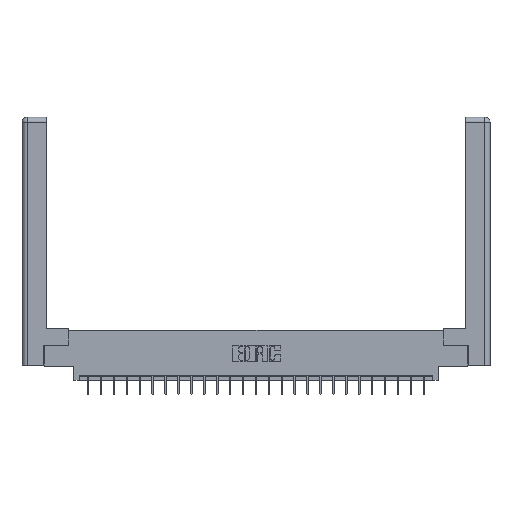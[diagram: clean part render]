
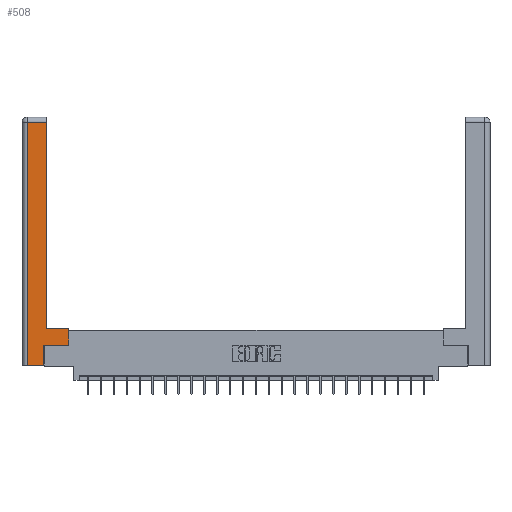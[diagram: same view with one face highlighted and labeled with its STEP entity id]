
A CAD part, top view. The second image highlights one B-rep face of the part: STEP entity #508.
In plain terms, the highlighted planar face has unit normal (0, 0, 1).
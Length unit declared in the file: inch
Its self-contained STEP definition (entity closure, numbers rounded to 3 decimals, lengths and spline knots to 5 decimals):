
#140 = FACE_OUTER_BOUND ( 'NONE', #25302, .T. ) ;
#165 = DIRECTION ( 'NONE',  ( 0., 1., 0. ) ) ;
#508 = ADVANCED_FACE ( 'NONE', ( #140 ), #7640, .F. ) ;
#1192 = ORIENTED_EDGE ( 'NONE', *, *, #4811, .T. ) ;
#1405 = DIRECTION ( 'NONE',  ( -1., 0., 0. ) ) ;
#1437 = ORIENTED_EDGE ( 'NONE', *, *, #23407, .T. ) ;
#1975 = LINE ( 'NONE', #7337, #19081 ) ;
#2334 = CARTESIAN_POINT ( 'NONE',  ( 0.0615, 0., 0. ) ) ;
#3073 = CARTESIAN_POINT ( 'NONE',  ( 0.295, 0.45, 0. ) ) ;
#4093 = CARTESIAN_POINT ( 'NONE',  ( 0.265, 0.245, 0. ) ) ;
#4225 = DIRECTION ( 'NONE',  ( 0., -1., 0. ) ) ;
#4312 = VERTEX_POINT ( 'NONE', #3073 ) ;
#4638 = VECTOR ( 'NONE', #24363, 39.37008 ) ;
#4811 = EDGE_CURVE ( 'NONE', #12248, #4312, #20631, .T. ) ;
#5860 = VECTOR ( 'NONE', #4225, 39.37008 ) ;
#6681 = ORIENTED_EDGE ( 'NONE', *, *, #22817, .T. ) ;
#6723 = VERTEX_POINT ( 'NONE', #22318 ) ;
#7089 = ORIENTED_EDGE ( 'NONE', *, *, #25089, .T. ) ;
#7107 = ORIENTED_EDGE ( 'NONE', *, *, #20207, .T. ) ;
#7214 = ORIENTED_EDGE ( 'NONE', *, *, #18998, .T. ) ;
#7253 = VECTOR ( 'NONE', #165, 39.37008 ) ;
#7297 = VECTOR ( 'NONE', #23084, 39.37008 ) ;
#7337 = CARTESIAN_POINT ( 'NONE',  ( 0.0615, 2.94, 0. ) ) ;
#7465 = CARTESIAN_POINT ( 'NONE',  ( 0.0615, 2.94, 0. ) ) ;
#7640 = PLANE ( 'NONE',  #12388 ) ;
#7835 = DIRECTION ( 'NONE',  ( 1., 0., 0. ) ) ;
#10400 = VERTEX_POINT ( 'NONE', #14519 ) ;
#10603 = VECTOR ( 'NONE', #7835, 39.37008 ) ;
#11315 = LINE ( 'NONE', #18001, #7253 ) ;
#11538 = ORIENTED_EDGE ( 'NONE', *, *, #19222, .T. ) ;
#11666 = CARTESIAN_POINT ( 'NONE',  ( 0., 0., 0. ) ) ;
#12248 = VERTEX_POINT ( 'NONE', #24705 ) ;
#12388 = AXIS2_PLACEMENT_3D ( 'NONE', #11666, #25491, #25231 ) ;
#13343 = VERTEX_POINT ( 'NONE', #7465 ) ;
#14519 = CARTESIAN_POINT ( 'NONE',  ( 0.265, 0., 0. ) ) ;
#14846 = VERTEX_POINT ( 'NONE', #20801 ) ;
#16338 = CARTESIAN_POINT ( 'NONE',  ( 0.265, 0., 0. ) ) ;
#16466 = LINE ( 'NONE', #2334, #5860 ) ;
#16989 = VECTOR ( 'NONE', #18937, 39.37008 ) ;
#17098 = LINE ( 'NONE', #21333, #18050 ) ;
#18001 = CARTESIAN_POINT ( 'NONE',  ( 0.565, 0.45, 0. ) ) ;
#18050 = VECTOR ( 'NONE', #24992, 39.37008 ) ;
#18194 = ORIENTED_EDGE ( 'NONE', *, *, #21734, .T. ) ;
#18791 = CARTESIAN_POINT ( 'NONE',  ( 0.295, 2.94, 0. ) ) ;
#18937 = DIRECTION ( 'NONE',  ( 0., 1., 0. ) ) ;
#18998 = EDGE_CURVE ( 'NONE', #6723, #10400, #19239, .T. ) ;
#19081 = VECTOR ( 'NONE', #1405, 39.37008 ) ;
#19222 = EDGE_CURVE ( 'NONE', #24564, #14846, #22371, .T. ) ;
#19239 = LINE ( 'NONE', #16338, #4638 ) ;
#19253 = CARTESIAN_POINT ( 'NONE',  ( 0.295, 3., 0. ) ) ;
#20178 = CARTESIAN_POINT ( 'NONE',  ( 0.565, 0.245, 0. ) ) ;
#20207 = EDGE_CURVE ( 'NONE', #13343, #6723, #16466, .T. ) ;
#20631 = LINE ( 'NONE', #23449, #7297 ) ;
#20801 = CARTESIAN_POINT ( 'NONE',  ( 0.565, 0.245, 0. ) ) ;
#21333 = CARTESIAN_POINT ( 'NONE',  ( 0.265, 0.245, 0. ) ) ;
#21734 = EDGE_CURVE ( 'NONE', #4312, #24817, #22226, .T. ) ;
#22226 = LINE ( 'NONE', #19253, #16989 ) ;
#22318 = CARTESIAN_POINT ( 'NONE',  ( 0.0615, 0., 0. ) ) ;
#22371 = LINE ( 'NONE', #20178, #10603 ) ;
#22817 = EDGE_CURVE ( 'NONE', #24817, #13343, #1975, .T. ) ;
#23084 = DIRECTION ( 'NONE',  ( -1., 0., 0. ) ) ;
#23407 = EDGE_CURVE ( 'NONE', #14846, #12248, #11315, .T. ) ;
#23449 = CARTESIAN_POINT ( 'NONE',  ( 0.295, 0.45, 0. ) ) ;
#24363 = DIRECTION ( 'NONE',  ( 1., 0., 0. ) ) ;
#24564 = VERTEX_POINT ( 'NONE', #4093 ) ;
#24705 = CARTESIAN_POINT ( 'NONE',  ( 0.565, 0.45, 0. ) ) ;
#24817 = VERTEX_POINT ( 'NONE', #18791 ) ;
#24992 = DIRECTION ( 'NONE',  ( 0., 1., 0. ) ) ;
#25089 = EDGE_CURVE ( 'NONE', #10400, #24564, #17098, .T. ) ;
#25231 = DIRECTION ( 'NONE',  ( -1., 0., 0. ) ) ;
#25302 = EDGE_LOOP ( 'NONE', ( #18194, #6681, #7107, #7214, #7089, #11538, #1437, #1192 ) ) ;
#25491 = DIRECTION ( 'NONE',  ( 0., 0., -1. ) ) ;
